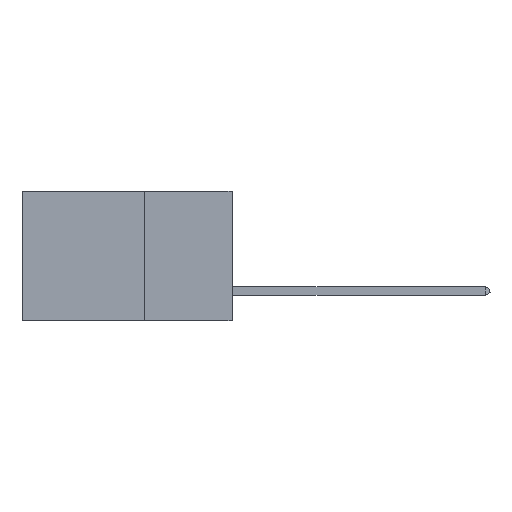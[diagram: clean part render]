
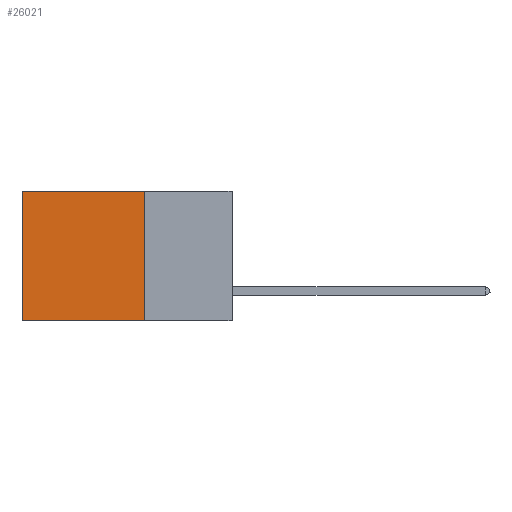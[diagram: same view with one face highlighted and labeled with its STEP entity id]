
A CAD part, left-side view. The second image highlights one B-rep face of the part: STEP entity #26021.
In plain terms, the highlighted planar face has unit normal (-1, 0, 0).
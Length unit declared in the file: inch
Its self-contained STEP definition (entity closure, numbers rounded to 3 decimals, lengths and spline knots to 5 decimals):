
#1284 = VECTOR ( 'NONE', #24623, 39.37008 ) ;
#1963 = AXIS2_PLACEMENT_3D ( 'NONE', #20707, #13585, #31631 ) ;
#3366 = PLANE ( 'NONE',  #1963 ) ;
#5961 = LINE ( 'NONE', #14531, #30392 ) ;
#6115 = VERTEX_POINT ( 'NONE', #17161 ) ;
#6650 = VECTOR ( 'NONE', #14497, 39.37008 ) ;
#7450 = CARTESIAN_POINT ( 'NONE',  ( 0.2875, 0.25, 0. ) ) ;
#7582 = CARTESIAN_POINT ( 'NONE',  ( 0.2875, 0.25, -0.37 ) ) ;
#8785 = CARTESIAN_POINT ( 'NONE',  ( 0.2875, 0.25, -0.37 ) ) ;
#9498 = ORIENTED_EDGE ( 'NONE', *, *, #26576, .F. ) ;
#10268 = VECTOR ( 'NONE', #40440, 39.37008 ) ;
#11250 = CARTESIAN_POINT ( 'NONE',  ( 0.2875, 0.6, 0. ) ) ;
#12016 = LINE ( 'NONE', #7450, #10268 ) ;
#12510 = EDGE_LOOP ( 'NONE', ( #15400, #9498, #23548, #38026 ) ) ;
#13585 = DIRECTION ( 'NONE',  ( 1., 0., 0. ) ) ;
#14497 = DIRECTION ( 'NONE',  ( 0., 0., -1. ) ) ;
#14531 = CARTESIAN_POINT ( 'NONE',  ( 0.2875, 0.25, 0. ) ) ;
#15400 = ORIENTED_EDGE ( 'NONE', *, *, #35267, .T. ) ;
#16028 = LINE ( 'NONE', #8785, #1284 ) ;
#17161 = CARTESIAN_POINT ( 'NONE',  ( 0.2875, 0.25, 0. ) ) ;
#20556 = FACE_OUTER_BOUND ( 'NONE', #12510, .T. ) ;
#20707 = CARTESIAN_POINT ( 'NONE',  ( 0.2875, 0.25, 0. ) ) ;
#21054 = VERTEX_POINT ( 'NONE', #27753 ) ;
#21946 = DIRECTION ( 'NONE',  ( 0., 1., 0. ) ) ;
#23548 = ORIENTED_EDGE ( 'NONE', *, *, #27348, .F. ) ;
#24623 = DIRECTION ( 'NONE',  ( 0., 1., 0. ) ) ;
#25660 = VERTEX_POINT ( 'NONE', #7582 ) ;
#26021 = ADVANCED_FACE ( 'NONE', ( #20556 ), #3366, .F. ) ;
#26576 = EDGE_CURVE ( 'NONE', #25660, #21054, #16028, .T. ) ;
#27348 = EDGE_CURVE ( 'NONE', #6115, #25660, #12016, .T. ) ;
#27753 = CARTESIAN_POINT ( 'NONE',  ( 0.2875, 0.6, -0.37 ) ) ;
#30392 = VECTOR ( 'NONE', #21946, 39.37008 ) ;
#30475 = VERTEX_POINT ( 'NONE', #11250 ) ;
#31631 = DIRECTION ( 'NONE',  ( 0., 0., -1. ) ) ;
#35267 = EDGE_CURVE ( 'NONE', #30475, #21054, #41855, .T. ) ;
#38026 = ORIENTED_EDGE ( 'NONE', *, *, #41786, .T. ) ;
#40440 = DIRECTION ( 'NONE',  ( 0., 0., -1. ) ) ;
#41786 = EDGE_CURVE ( 'NONE', #6115, #30475, #5961, .T. ) ;
#41855 = LINE ( 'NONE', #46715, #6650 ) ;
#46715 = CARTESIAN_POINT ( 'NONE',  ( 0.2875, 0.6, 0. ) ) ;
